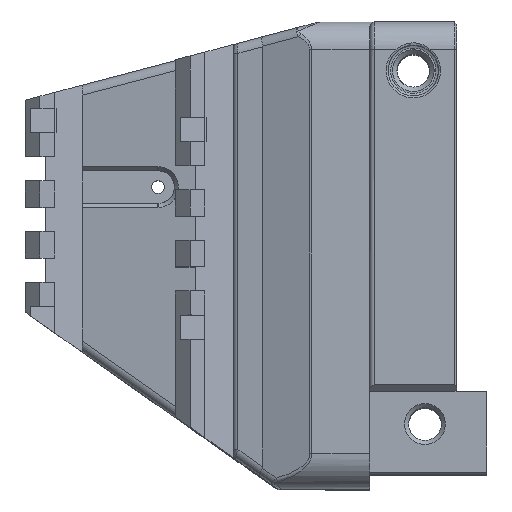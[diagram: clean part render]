
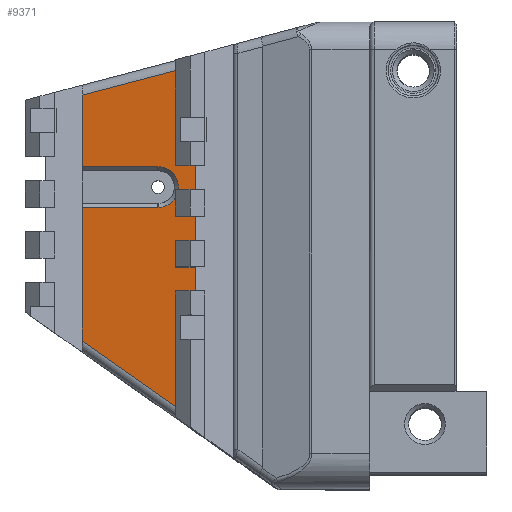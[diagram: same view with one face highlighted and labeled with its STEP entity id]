
A CAD part, top view. The second image highlights one B-rep face of the part: STEP entity #9371.
In plain terms, the highlighted planar face has unit normal (-0.138, 0, 0.99).
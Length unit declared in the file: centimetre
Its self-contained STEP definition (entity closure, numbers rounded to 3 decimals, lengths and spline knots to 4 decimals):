
#98=B_SPLINE_CURVE_WITH_KNOTS($,3,(#17079,#17080,#17081,#17082,#17083,#17084,
#17085,#17086),.UNSPECIFIED.,.F.,.F.,(4,1,1,1,1,4),(-1.5708,-0.6732,
0.2244,0.6732,1.122,1.5708),
 .UNSPECIFIED.);
#955=LINE($,#17042,#1831);
#958=LINE($,#17121,#1834);
#960=LINE($,#17131,#1836);
#963=LINE($,#17151,#1839);
#964=LINE($,#17158,#1840);
#965=LINE($,#17160,#1841);
#966=LINE($,#17162,#1842);
#967=LINE($,#17164,#1843);
#968=LINE($,#17165,#1844);
#1831=VECTOR($,#12222,1.5034);
#1834=VECTOR($,#12225,0.0112);
#1836=VECTOR($,#12229,1.5034);
#1839=VECTOR($,#12232,0.0112);
#1840=VECTOR($,#12235,2.6491);
#1841=VECTOR($,#12236,4.4048);
#1842=VECTOR($,#12237,8.3386);
#1843=VECTOR($,#12238,3.7355);
#1844=VECTOR($,#12239,1.4202);
#2309=PLANE($,#10126);
#3004=FACE_OUTER_BOUND($,#3642,.T.);
#3642=EDGE_LOOP($,(#8171,#8172,#8173,#8174,#8175,#8176,#8177,#8178,#8179,
#8180));
#4732=VERTEX_POINT($,#17035);
#4735=VERTEX_POINT($,#17040);
#4737=VERTEX_POINT($,#17076);
#4738=VERTEX_POINT($,#17078);
#4741=VERTEX_POINT($,#17128);
#4742=VERTEX_POINT($,#17130);
#4744=VERTEX_POINT($,#17157);
#4745=VERTEX_POINT($,#17159);
#4746=VERTEX_POINT($,#17161);
#4747=VERTEX_POINT($,#17163);
#5920=EDGE_CURVE($,#4735,#4732,#955,.T.);
#5922=EDGE_CURVE($,#4737,#4738,#98,.T.);
#5925=EDGE_CURVE($,#4738,#4735,#958,.T.);
#5928=EDGE_CURVE($,#4741,#4742,#960,.T.);
#5931=EDGE_CURVE($,#4742,#4737,#963,.T.);
#5933=EDGE_CURVE($,#4744,#4741,#964,.T.);
#5934=EDGE_CURVE($,#4745,#4744,#965,.T.);
#5935=EDGE_CURVE($,#4745,#4746,#966,.F.);
#5936=EDGE_CURVE($,#4747,#4746,#967,.T.);
#5937=EDGE_CURVE($,#4732,#4747,#968,.T.);
#8171=ORIENTED_EDGE($,*,*,#5920,.F.);
#8172=ORIENTED_EDGE($,*,*,#5925,.F.);
#8173=ORIENTED_EDGE($,*,*,#5922,.F.);
#8174=ORIENTED_EDGE($,*,*,#5931,.F.);
#8175=ORIENTED_EDGE($,*,*,#5928,.F.);
#8176=ORIENTED_EDGE($,*,*,#5933,.F.);
#8177=ORIENTED_EDGE($,*,*,#5934,.F.);
#8178=ORIENTED_EDGE($,*,*,#5935,.T.);
#8179=ORIENTED_EDGE($,*,*,#5936,.F.);
#8180=ORIENTED_EDGE($,*,*,#5937,.F.);
#9371=ADVANCED_FACE($,(#3004),#2309,.F.);
#10126=AXIS2_PLACEMENT_3D($,#17156,#12233,#12234);
#12222=DIRECTION($,(-0.99,0.,-0.138));
#12225=DIRECTION($,(-0.99,0.,-0.138));
#12229=DIRECTION($,(0.99,0.,0.138));
#12232=DIRECTION($,(0.99,0.,0.138));
#12233=DIRECTION('center_axis',(0.138,0.,
-0.99));
#12234=DIRECTION('ref_axis',(-0.99,0.,
-0.138));
#12235=DIRECTION($,(0.,1.,0.));
#12236=DIRECTION($,(-0.813,0.571,-0.114));
#12237=DIRECTION($,(0.,-1.,0.));
#12238=DIRECTION($,(0.958,0.252,0.134));
#12239=DIRECTION($,(0.,1.,0.));
#17035=CARTESIAN_POINT('',(-25.2982,5.0571,-8.65));
#17040=CARTESIAN_POINT('',(-23.8093,5.0571,-8.4421));
#17042=CARTESIAN_POINT($,(-24.9981,5.0571,-8.6081));
#17076=CARTESIAN_POINT('',(-23.7982,4.2471,-8.4405));
#17078=CARTESIAN_POINT('',(-23.7982,5.0571,-8.4405));
#17079=CARTESIAN_POINT('Ctrl Pts',(-23.7982,4.2471,-8.4405));
#17080=CARTESIAN_POINT('Ctrl Pts',(-23.6775,4.2471,-8.4236));
#17081=CARTESIAN_POINT('Ctrl Pts',(-23.4367,4.3635,-8.39));
#17082=CARTESIAN_POINT('Ctrl Pts',(-23.3622,4.6897,-8.3796));
#17083=CARTESIAN_POINT('Ctrl Pts',(-23.4719,4.9138,-8.3949));
#17084=CARTESIAN_POINT('Ctrl Pts',(-23.6169,5.0296,-8.4152));
#17085=CARTESIAN_POINT('Ctrl Pts',(-23.7378,5.0571,-8.4321));
#17086=CARTESIAN_POINT('Ctrl Pts',(-23.7982,5.0571,-8.4405));
#17121=CARTESIAN_POINT($,(-23.7982,5.0571,-8.4405));
#17128=CARTESIAN_POINT('',(-25.2982,4.2471,-8.65));
#17130=CARTESIAN_POINT('',(-23.8093,4.2471,-8.4421));
#17131=CARTESIAN_POINT($,(-24.9981,4.2471,-8.6081));
#17151=CARTESIAN_POINT($,(-23.8093,4.2471,-8.4421));
#17156=CARTESIAN_POINT('Origin',(-26.2886,-1.3536,-8.7883));
#17157=CARTESIAN_POINT('',(-25.2982,1.598,-8.65));
#17158=CARTESIAN_POINT($,(-25.2982,1.7147,-8.65));
#17159=CARTESIAN_POINT('',(-21.7182,-0.9191,-8.15));
#17160=CARTESIAN_POINT($,(-26.5173,2.4552,-8.8203));
#17161=CARTESIAN_POINT('',(-21.7182,7.4194,-8.15));
#17162=CARTESIAN_POINT($,(-21.7182,-1.3536,-8.15));
#17163=CARTESIAN_POINT('',(-25.2982,6.4773,-8.65));
#17164=CARTESIAN_POINT($,(-27.2555,5.9623,-8.9234));
#17165=CARTESIAN_POINT($,(-25.2982,1.7147,-8.65));
